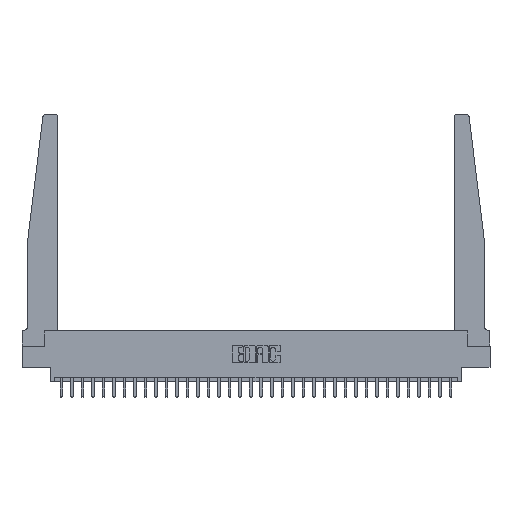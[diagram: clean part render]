
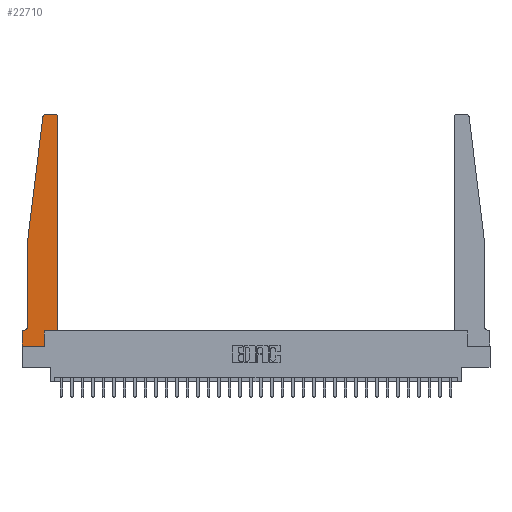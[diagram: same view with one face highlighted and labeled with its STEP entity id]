
A CAD part, top view. The second image highlights one B-rep face of the part: STEP entity #22710.
In plain terms, the highlighted planar face has unit normal (0, 0, 1).
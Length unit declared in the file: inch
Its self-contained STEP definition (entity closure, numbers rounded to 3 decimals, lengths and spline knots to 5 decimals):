
#267 = DIRECTION ( 'NONE',  ( -1., 0., 0. ) ) ;
#411 = CARTESIAN_POINT ( 'NONE',  ( 0.065, 0.2375, 0.37 ) ) ;
#1094 = VECTOR ( 'NONE', #18309, 39.37008 ) ;
#1095 = VERTEX_POINT ( 'NONE', #2826 ) ;
#1439 = VECTOR ( 'NONE', #14961, 39.37008 ) ;
#2123 = ORIENTED_EDGE ( 'NONE', *, *, #13835, .T. ) ;
#2450 = LINE ( 'NONE', #19186, #26589 ) ;
#2471 = DIRECTION ( 'NONE',  ( 0., 0., -1. ) ) ;
#2619 = ORIENTED_EDGE ( 'NONE', *, *, #8854, .T. ) ;
#2694 = LINE ( 'NONE', #24037, #1439 ) ;
#2826 = CARTESIAN_POINT ( 'NONE',  ( 0.015, 0.1875, 0.37 ) ) ;
#3113 = EDGE_LOOP ( 'NONE', ( #17887, #14535, #30704, #7202, #14669, #19990, #21539, #2619, #27612, #9434, #14172, #2123 ) ) ;
#3250 = CARTESIAN_POINT ( 'NONE',  ( 0., 0.1875, 0.37 ) ) ;
#3354 = DIRECTION ( 'NONE',  ( 0., 0., 1. ) ) ;
#3597 = LINE ( 'NONE', #30119, #1094 ) ;
#5399 = FACE_OUTER_BOUND ( 'NONE', #3113, .T. ) ;
#5548 = DIRECTION ( 'NONE',  ( 0., 0., 1. ) ) ;
#5811 = VERTEX_POINT ( 'NONE', #13447 ) ;
#5966 = VECTOR ( 'NONE', #6578, 39.37008 ) ;
#6093 = CARTESIAN_POINT ( 'NONE',  ( 0.395, 2.72, 0.37 ) ) ;
#6223 = LINE ( 'NONE', #6529, #18273 ) ;
#6358 = CARTESIAN_POINT ( 'NONE',  ( 0.2605, 0.18, 0.37 ) ) ;
#6529 = CARTESIAN_POINT ( 'NONE',  ( 0.065, 1.25, 0.37 ) ) ;
#6578 = DIRECTION ( 'NONE',  ( 0., 1., 0. ) ) ;
#6723 = DIRECTION ( 'NONE',  ( 0., 0., 1. ) ) ;
#7202 = ORIENTED_EDGE ( 'NONE', *, *, #29813, .T. ) ;
#7331 = VECTOR ( 'NONE', #9756, 39.37008 ) ;
#7399 = CARTESIAN_POINT ( 'NONE',  ( 0.425, 0.18, 0.37 ) ) ;
#7585 = DIRECTION ( 'NONE',  ( 1., 0., 0. ) ) ;
#7672 = CARTESIAN_POINT ( 'NONE',  ( 0.065, 1.25, 0.37 ) ) ;
#7675 = LINE ( 'NONE', #26710, #27688 ) ;
#7710 = VERTEX_POINT ( 'NONE', #12055 ) ;
#7904 = CARTESIAN_POINT ( 'NONE',  ( 0.395, 2.75, 0.37 ) ) ;
#8189 = CARTESIAN_POINT ( 'NONE',  ( 0., 0.1875, 0.37 ) ) ;
#8659 = CARTESIAN_POINT ( 'NONE',  ( 0.24675, 2.72367, 0.37 ) ) ;
#8854 = EDGE_CURVE ( 'NONE', #11133, #30738, #7675, .T. ) ;
#9434 = ORIENTED_EDGE ( 'NONE', *, *, #11937, .T. ) ;
#9756 = DIRECTION ( 'NONE',  ( 1., 0., 0. ) ) ;
#10694 = EDGE_CURVE ( 'NONE', #15279, #17352, #6223, .T. ) ;
#10979 = EDGE_CURVE ( 'NONE', #18232, #1095, #30705, .T. ) ;
#11133 = VERTEX_POINT ( 'NONE', #24480 ) ;
#11508 = EDGE_CURVE ( 'NONE', #30738, #19086, #13029, .T. ) ;
#11594 = EDGE_CURVE ( 'NONE', #16196, #15279, #25262, .T. ) ;
#11937 = EDGE_CURVE ( 'NONE', #19086, #7710, #21637, .T. ) ;
#12055 = CARTESIAN_POINT ( 'NONE',  ( 0.425, 0.18, 0.37 ) ) ;
#12500 = VERTEX_POINT ( 'NONE', #3250 ) ;
#12713 = EDGE_CURVE ( 'NONE', #23393, #16196, #19020, .T. ) ;
#13029 = LINE ( 'NONE', #22275, #22778 ) ;
#13339 = VECTOR ( 'NONE', #16830, 39.37008 ) ;
#13447 = CARTESIAN_POINT ( 'NONE',  ( 0.425, 2.72, 0.37 ) ) ;
#13835 = EDGE_CURVE ( 'NONE', #5811, #23393, #17804, .T. ) ;
#14172 = ORIENTED_EDGE ( 'NONE', *, *, #26992, .T. ) ;
#14353 = CARTESIAN_POINT ( 'NONE',  ( 0.015, 0.2375, 0.37 ) ) ;
#14535 = ORIENTED_EDGE ( 'NONE', *, *, #11594, .T. ) ;
#14669 = ORIENTED_EDGE ( 'NONE', *, *, #10979, .T. ) ;
#14961 = DIRECTION ( 'NONE',  ( 0., -1., 0. ) ) ;
#15279 = VERTEX_POINT ( 'NONE', #8659 ) ;
#15301 = AXIS2_PLACEMENT_3D ( 'NONE', #6093, #6723, #25140 ) ;
#15750 = DIRECTION ( 'NONE',  ( -0.122, -0.992, 0. ) ) ;
#16196 = VERTEX_POINT ( 'NONE', #22341 ) ;
#16437 = EDGE_CURVE ( 'NONE', #12500, #11133, #2694, .T. ) ;
#16753 = DIRECTION ( 'NONE',  ( 1., 0., 0. ) ) ;
#16830 = DIRECTION ( 'NONE',  ( -1., 0., 0. ) ) ;
#17352 = VERTEX_POINT ( 'NONE', #7672 ) ;
#17735 = DIRECTION ( 'NONE',  ( 0., 1., 0. ) ) ;
#17804 = CIRCLE ( 'NONE', #15301, 0.03 ) ;
#17887 = ORIENTED_EDGE ( 'NONE', *, *, #12713, .T. ) ;
#18232 = VERTEX_POINT ( 'NONE', #411 ) ;
#18273 = VECTOR ( 'NONE', #15750, 39.37008 ) ;
#18309 = DIRECTION ( 'NONE',  ( 0., -1., 0. ) ) ;
#19020 = LINE ( 'NONE', #28500, #13339 ) ;
#19086 = VERTEX_POINT ( 'NONE', #6358 ) ;
#19186 = CARTESIAN_POINT ( 'NONE',  ( 0.065, 0.1875, 0.37 ) ) ;
#19990 = ORIENTED_EDGE ( 'NONE', *, *, #23286, .T. ) ;
#20816 = LINE ( 'NONE', #30282, #5966 ) ;
#21539 = ORIENTED_EDGE ( 'NONE', *, *, #16437, .T. ) ;
#21550 = DIRECTION ( 'NONE',  ( -1., 0., 0. ) ) ;
#21637 = LINE ( 'NONE', #7399, #7331 ) ;
#22275 = CARTESIAN_POINT ( 'NONE',  ( 0.2605, 0.18, 0.37 ) ) ;
#22341 = CARTESIAN_POINT ( 'NONE',  ( 0.27653, 2.75, 0.37 ) ) ;
#22710 = ADVANCED_FACE ( 'NONE', ( #5399 ), #29100, .T. ) ;
#22778 = VECTOR ( 'NONE', #17735, 39.37008 ) ;
#23286 = EDGE_CURVE ( 'NONE', #1095, #12500, #2450, .T. ) ;
#23393 = VERTEX_POINT ( 'NONE', #7904 ) ;
#24037 = CARTESIAN_POINT ( 'NONE',  ( 0., 0., 0.37 ) ) ;
#24480 = CARTESIAN_POINT ( 'NONE',  ( 0., 0., 0.37 ) ) ;
#24752 = CARTESIAN_POINT ( 'NONE',  ( 0.27653, 2.72, 0.37 ) ) ;
#25072 = AXIS2_PLACEMENT_3D ( 'NONE', #8189, #5548, #7585 ) ;
#25140 = DIRECTION ( 'NONE',  ( 1., 0., 0. ) ) ;
#25262 = CIRCLE ( 'NONE', #29232, 0.03 ) ;
#25740 = AXIS2_PLACEMENT_3D ( 'NONE', #14353, #2471, #21550 ) ;
#26589 = VECTOR ( 'NONE', #267, 39.37008 ) ;
#26710 = CARTESIAN_POINT ( 'NONE',  ( 0., 0., 0.37 ) ) ;
#26992 = EDGE_CURVE ( 'NONE', #7710, #5811, #20816, .T. ) ;
#27241 = CARTESIAN_POINT ( 'NONE',  ( 0.2605, 0., 0.37 ) ) ;
#27612 = ORIENTED_EDGE ( 'NONE', *, *, #11508, .T. ) ;
#27688 = VECTOR ( 'NONE', #16753, 39.37008 ) ;
#28500 = CARTESIAN_POINT ( 'NONE',  ( 0.25, 2.75, 0.37 ) ) ;
#29100 = PLANE ( 'NONE',  #25072 ) ;
#29232 = AXIS2_PLACEMENT_3D ( 'NONE', #24752, #3354, #29554 ) ;
#29554 = DIRECTION ( 'NONE',  ( 1., 0., 0. ) ) ;
#29813 = EDGE_CURVE ( 'NONE', #17352, #18232, #3597, .T. ) ;
#30119 = CARTESIAN_POINT ( 'NONE',  ( 0.065, 1.25, 0.37 ) ) ;
#30282 = CARTESIAN_POINT ( 'NONE',  ( 0.425, 0.18, 0.37 ) ) ;
#30704 = ORIENTED_EDGE ( 'NONE', *, *, #10694, .T. ) ;
#30705 = CIRCLE ( 'NONE', #25740, 0.05 ) ;
#30738 = VERTEX_POINT ( 'NONE', #27241 ) ;
